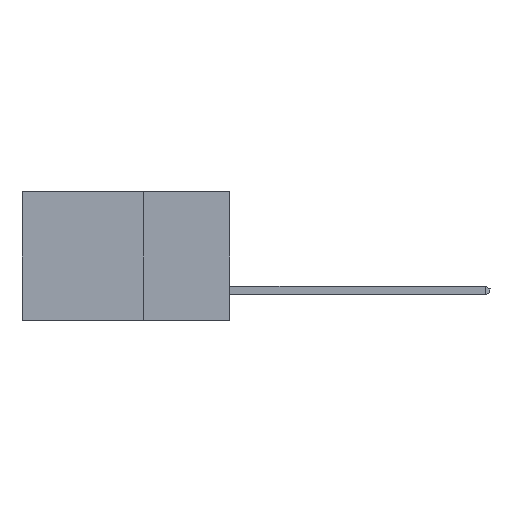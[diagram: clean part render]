
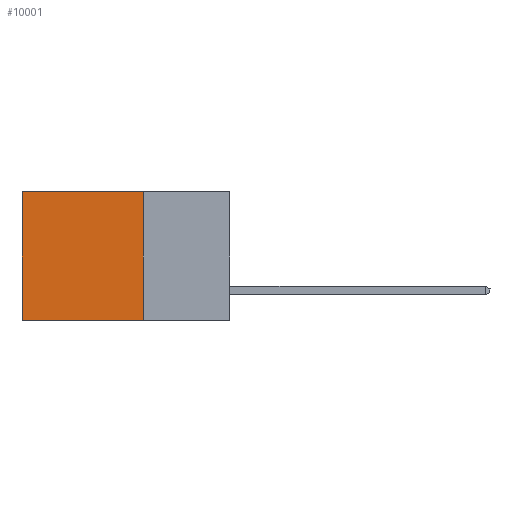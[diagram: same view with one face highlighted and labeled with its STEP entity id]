
A CAD part, left-side view. The second image highlights one B-rep face of the part: STEP entity #10001.
In plain terms, the highlighted planar face has unit normal (-1, 0, 0).
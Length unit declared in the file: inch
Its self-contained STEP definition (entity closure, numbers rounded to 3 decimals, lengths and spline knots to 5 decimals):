
#676 = CARTESIAN_POINT ( 'NONE',  ( 0.2615, 0.25, -0.37 ) ) ;
#1483 = EDGE_LOOP ( 'NONE', ( #7207, #10826, #19022, #18859 ) ) ;
#1482 = CARTESIAN_POINT ( 'NONE',  ( 0.2615, 0.25, 0. ) ) ;
#2233 = EDGE_CURVE ( 'NONE', #13054, #19176, #8711, .T. ) ;
#2414 = CARTESIAN_POINT ( 'NONE',  ( 0.2615, 0.25, -0.37 ) ) ;
#3013 = AXIS2_PLACEMENT_3D ( 'NONE', #17770, #16567, #19667 ) ;
#4173 = DIRECTION ( 'NONE',  ( 0., 0., -1. ) ) ;
#4714 = VECTOR ( 'NONE', #4173, 39.37008 ) ;
#5712 = CARTESIAN_POINT ( 'NONE',  ( 0.2615, 0.25, 0. ) ) ;
#6530 = CARTESIAN_POINT ( 'NONE',  ( 0.2615, 0.6, -0.37 ) ) ;
#6668 = EDGE_CURVE ( 'NONE', #19176, #17928, #11651, .T. ) ;
#7207 = ORIENTED_EDGE ( 'NONE', *, *, #6668, .T. ) ;
#7287 = FACE_OUTER_BOUND ( 'NONE', #1483, .T. ) ;
#8150 = CARTESIAN_POINT ( 'NONE',  ( 0.2615, 0.25, -0.37 ) ) ;
#8207 = DIRECTION ( 'NONE',  ( 0., 1., 0. ) ) ;
#8374 = DIRECTION ( 'NONE',  ( 0., 0., -1. ) ) ;
#8711 = LINE ( 'NONE', #5712, #11293 ) ;
#10001 = ADVANCED_FACE ( 'NONE', ( #7287 ), #10389, .F. ) ;
#10389 = PLANE ( 'NONE',  #3013 ) ;
#10826 = ORIENTED_EDGE ( 'NONE', *, *, #13987, .F. ) ;
#11293 = VECTOR ( 'NONE', #17889, 39.37008 ) ;
#11651 = LINE ( 'NONE', #17537, #4714 ) ;
#13054 = VERTEX_POINT ( 'NONE', #1482 ) ;
#13830 = CARTESIAN_POINT ( 'NONE',  ( 0.2615, 0.6, 0. ) ) ;
#13987 = EDGE_CURVE ( 'NONE', #17546, #17928, #17280, .T. ) ;
#15747 = LINE ( 'NONE', #676, #17803 ) ;
#16567 = DIRECTION ( 'NONE',  ( 1., 0., 0. ) ) ;
#17123 = EDGE_CURVE ( 'NONE', #13054, #17546, #15747, .T. ) ;
#17280 = LINE ( 'NONE', #2414, #19365 ) ;
#17537 = CARTESIAN_POINT ( 'NONE',  ( 0.2615, 0.6, -0.37 ) ) ;
#17546 = VERTEX_POINT ( 'NONE', #8150 ) ;
#17770 = CARTESIAN_POINT ( 'NONE',  ( 0.2615, 0.25, -0.37 ) ) ;
#17803 = VECTOR ( 'NONE', #8374, 39.37008 ) ;
#17889 = DIRECTION ( 'NONE',  ( 0., 1., 0. ) ) ;
#17928 = VERTEX_POINT ( 'NONE', #6530 ) ;
#18859 = ORIENTED_EDGE ( 'NONE', *, *, #2233, .T. ) ;
#19022 = ORIENTED_EDGE ( 'NONE', *, *, #17123, .F. ) ;
#19176 = VERTEX_POINT ( 'NONE', #13830 ) ;
#19365 = VECTOR ( 'NONE', #8207, 39.37008 ) ;
#19667 = DIRECTION ( 'NONE',  ( 0., 0., -1. ) ) ;
